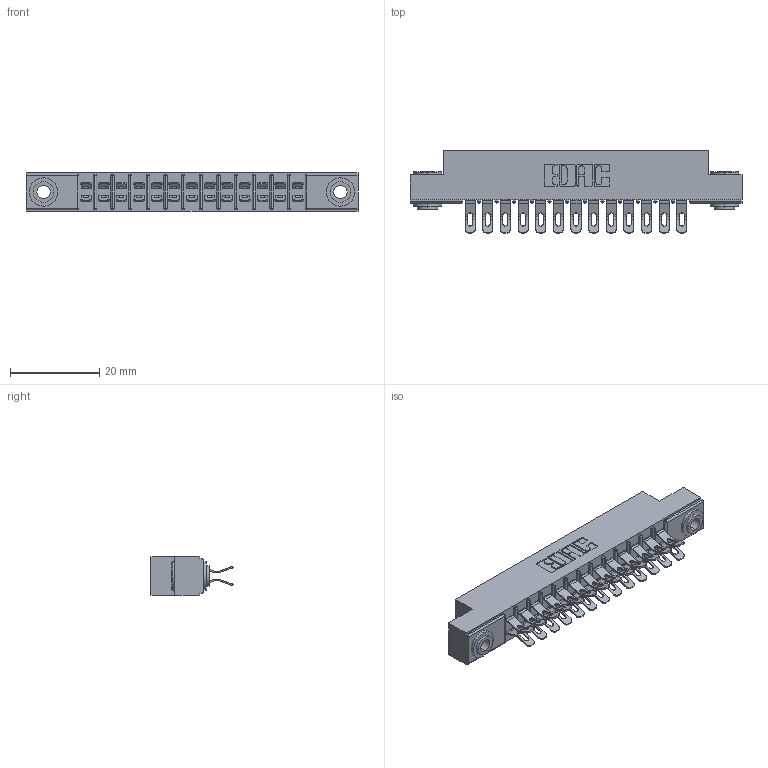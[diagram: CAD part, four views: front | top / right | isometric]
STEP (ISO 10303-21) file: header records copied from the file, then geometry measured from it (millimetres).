
FILE_DESCRIPTION (( 'STEP AP203' ), '1' );
FILE_NAME ('305-026-555-503.STEP', '2019-09-09T15:20:45', ( '' ), ( '' ), 'SwSTEP 2.0', 'SolidWorks 2016', '' );
FILE_SCHEMA (( 'CONFIG_CONTROL_DESIGN' ));
Length unit declared in the file: inch
Products named in the file (4): 305-026-555-503; 345-250-002_345-250-002-102; 305 Part_.156 Dia; 305-290-001_555
Assembly tree (29 placements, depth 2):
  305-026-555-503
    305 Part_.156 Dia
    305-290-001_555  x26
    345-250-002_345-250-002-102  x2
Bounding box: 74.52 x 18.41 x 8.71 mm (x, y, z)
Volume: 4579.4 mm3; surface area: 9226.5 mm2
Topology: 29 solids, 29 shells, 1884 faces, 5563 edges, 3634 vertices
Faces by surface type: plane 924, cylinder 900, sphere 52, cone 8
Entity records: 19295 total; most frequent: CARTESIAN_POINT 3192, ORIENTED_EDGE 3146, DIRECTION 3121, EDGE_CURVE 1573, VECTOR 1211, LINE 1211, VERTEX_POINT 1010, AXIS2_PLACEMENT_3D 955
